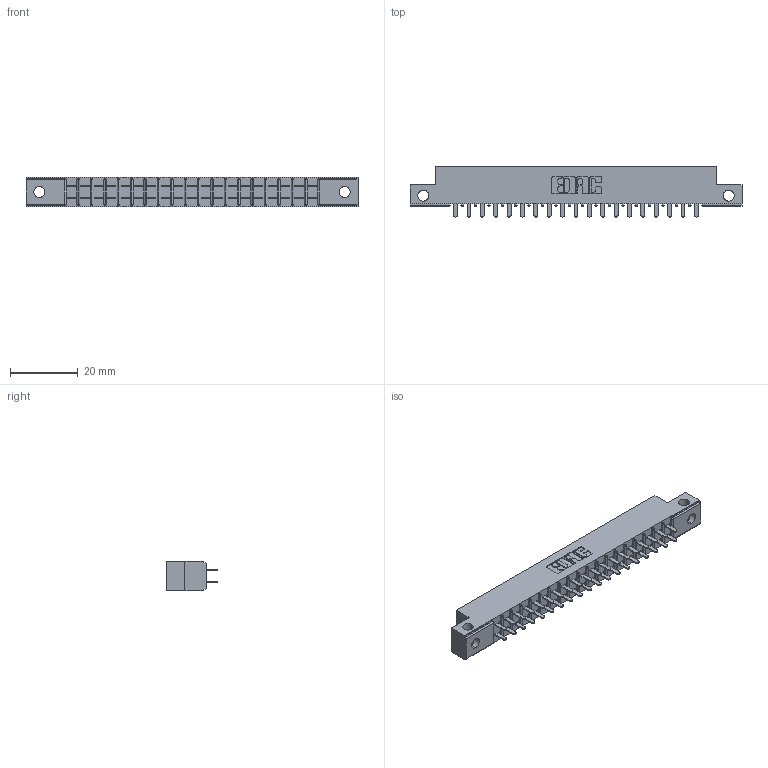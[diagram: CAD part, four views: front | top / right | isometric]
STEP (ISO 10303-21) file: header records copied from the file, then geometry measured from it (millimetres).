
FILE_DESCRIPTION (( 'STEP AP203' ), '1' );
FILE_NAME ('315-038-521-212.STEP', '2020-09-20T02:34:42', ( '' ), ( '' ), 'SwSTEP 2.0', 'SolidWorks 2020', '' );
FILE_SCHEMA (( 'CONFIG_CONTROL_DESIGN' ));
Length unit declared in the file: inch
Products named in the file (3): 315-038-521-212; 305-290-001_521; 305 Part_.128 Dia
Assembly tree (39 placements, depth 2):
  315-038-521-212
    305 Part_.128 Dia
    305-290-001_521  x38
Bounding box: 98.3 x 14.86 x 8.71 mm (x, y, z)
Volume: 6002.7 mm3; surface area: 10983 mm2
Topology: 39 solids, 39 shells, 1876 faces, 5349 edges, 3458 vertices
Faces by surface type: plane 1094, cylinder 706, sphere 76
Entity records: 23658 total; most frequent: CARTESIAN_POINT 3963, ORIENTED_EDGE 3886, DIRECTION 3791, EDGE_CURVE 1943, LINE 1531, VECTOR 1531, VERTEX_POINT 1238, AXIS2_PLACEMENT_3D 1130
